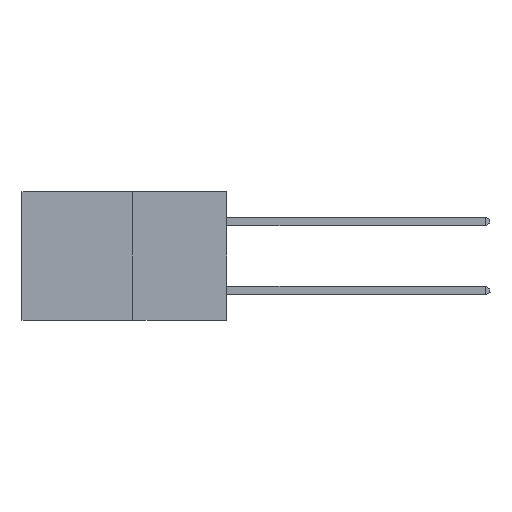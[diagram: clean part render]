
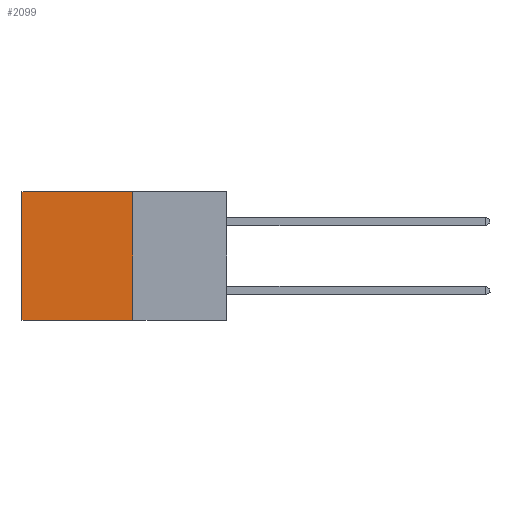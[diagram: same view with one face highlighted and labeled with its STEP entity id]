
A CAD part, left-side view. The second image highlights one B-rep face of the part: STEP entity #2099.
In plain terms, the highlighted planar face has unit normal (-1, 0, 0).
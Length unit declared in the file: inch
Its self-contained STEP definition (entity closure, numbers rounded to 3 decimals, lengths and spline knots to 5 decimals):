
#62 = DIRECTION ( 'NONE',  ( 0., 1., 0. ) ) ;
#228 = EDGE_CURVE ( 'NONE', #7250, #2511, #651, .T. ) ;
#343 = CARTESIAN_POINT ( 'NONE',  ( 0.277, 0.27, -0.37 ) ) ;
#345 = ORIENTED_EDGE ( 'NONE', *, *, #1321, .F. ) ;
#365 = LINE ( 'NONE', #4008, #4183 ) ;
#391 = EDGE_CURVE ( 'NONE', #2511, #5883, #3730, .T. ) ;
#651 = LINE ( 'NONE', #7347, #2304 ) ;
#1321 = EDGE_CURVE ( 'NONE', #6305, #5883, #365, .T. ) ;
#1337 = LINE ( 'NONE', #343, #6808 ) ;
#1664 = EDGE_CURVE ( 'NONE', #7250, #6305, #1337, .T. ) ;
#1769 = DIRECTION ( 'NONE',  ( 0., 0., -1. ) ) ;
#2000 = DIRECTION ( 'NONE',  ( 0., 0., -1. ) ) ;
#2099 = ADVANCED_FACE ( 'NONE', ( #8847 ), #6043, .F. ) ;
#2194 = AXIS2_PLACEMENT_3D ( 'NONE', #6765, #3509, #1769 ) ;
#2304 = VECTOR ( 'NONE', #5330, 39.37008 ) ;
#2511 = VERTEX_POINT ( 'NONE', #8722 ) ;
#2926 = ORIENTED_EDGE ( 'NONE', *, *, #391, .T. ) ;
#3509 = DIRECTION ( 'NONE',  ( 1., 0., 0. ) ) ;
#3730 = LINE ( 'NONE', #8962, #5235 ) ;
#4008 = CARTESIAN_POINT ( 'NONE',  ( 0.277, 0.27, -0.37 ) ) ;
#4183 = VECTOR ( 'NONE', #62, 39.37008 ) ;
#4305 = CARTESIAN_POINT ( 'NONE',  ( 0.277, 0.27, -0.37 ) ) ;
#4760 = ORIENTED_EDGE ( 'NONE', *, *, #1664, .F. ) ;
#5235 = VECTOR ( 'NONE', #6242, 39.37008 ) ;
#5330 = DIRECTION ( 'NONE',  ( 0., 1., 0. ) ) ;
#5718 = CARTESIAN_POINT ( 'NONE',  ( 0.277, 0.59, -0.37 ) ) ;
#5883 = VERTEX_POINT ( 'NONE', #5718 ) ;
#6043 = PLANE ( 'NONE',  #2194 ) ;
#6242 = DIRECTION ( 'NONE',  ( 0., 0., -1. ) ) ;
#6305 = VERTEX_POINT ( 'NONE', #4305 ) ;
#6490 = ORIENTED_EDGE ( 'NONE', *, *, #228, .T. ) ;
#6765 = CARTESIAN_POINT ( 'NONE',  ( 0.277, 0.27, -0.37 ) ) ;
#6808 = VECTOR ( 'NONE', #2000, 39.37008 ) ;
#7250 = VERTEX_POINT ( 'NONE', #7354 ) ;
#7347 = CARTESIAN_POINT ( 'NONE',  ( 0.277, 0.27, 0. ) ) ;
#7354 = CARTESIAN_POINT ( 'NONE',  ( 0.277, 0.27, 0. ) ) ;
#8230 = EDGE_LOOP ( 'NONE', ( #2926, #345, #4760, #6490 ) ) ;
#8722 = CARTESIAN_POINT ( 'NONE',  ( 0.277, 0.59, 0. ) ) ;
#8847 = FACE_OUTER_BOUND ( 'NONE', #8230, .T. ) ;
#8962 = CARTESIAN_POINT ( 'NONE',  ( 0.277, 0.59, -0.37 ) ) ;
